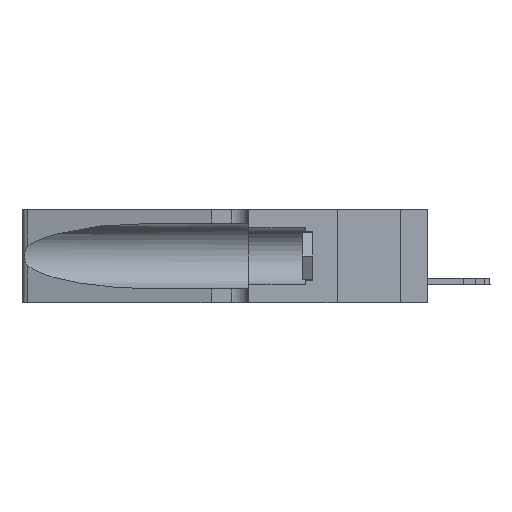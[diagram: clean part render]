
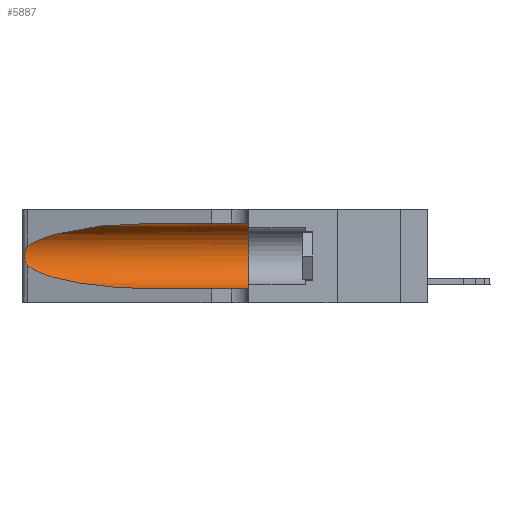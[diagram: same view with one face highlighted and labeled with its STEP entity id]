
A CAD part, left-side view. The second image highlights one B-rep face of the part: STEP entity #5887.
In plain terms, the highlighted cylindrical face has radius 3.308 mm (diameter 6.617 mm), a partial arc.
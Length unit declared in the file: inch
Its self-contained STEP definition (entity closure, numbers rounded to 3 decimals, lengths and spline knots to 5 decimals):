
#443 = FACE_OUTER_BOUND ( 'NONE', #18320, .T. ) ;
#533 = B_SPLINE_CURVE_WITH_KNOTS ( 'NONE', 3,
 ( #10524, #19248, #7877, #2828, #20661, #9650, #4468, #19108, #3426, #19643, #11725, #555, #16624, #3634 ),
 .UNSPECIFIED., .F., .F.,
 ( 4, 2, 2, 2, 2, 2, 4 ),
 ( 0., 0.00027, 0.00053, 0.00107, 0.0016, 0.00187, 0.00214 ),
 .UNSPECIFIED. ) ;
#555 = CARTESIAN_POINT ( 'NONE',  ( 0.25639, 1.23186, 0.15144 ) ) ;
#706 = CARTESIAN_POINT ( 'NONE',  ( 0.1305, 0.35, 0.185 ) ) ;
#826 = CARTESIAN_POINT ( 'NONE',  ( 0.1305, 0.72297, 0.05475 ) ) ;
#1690 = CIRCLE ( 'NONE', #1766, 0.13025 ) ;
#1766 = AXIS2_PLACEMENT_3D ( 'NONE', #706, #6352, #19618 ) ;
#1931 = LINE ( 'NONE', #5528, #7491 ) ;
#2828 = CARTESIAN_POINT ( 'NONE',  ( 0.25787, 1.23484, 0.2124 ) ) ;
#3426 = CARTESIAN_POINT ( 'NONE',  ( 0.26017, 1.23833, 0.17102 ) ) ;
#3464 = LINE ( 'NONE', #11767, #13092 ) ;
#3634 = CARTESIAN_POINT ( 'NONE',  ( 0.25487, 1.22718, 0.14631 ) ) ;
#3800 = EDGE_CURVE ( 'NONE', #15225, #18798, #4945, .T. ) ;
#4468 = CARTESIAN_POINT ( 'NONE',  ( 0.26075, 1.23896, 0.19203 ) ) ;
#4945 =( BOUNDED_CURVE ( )  B_SPLINE_CURVE ( 3, ( #10386, #12267, #8804, #20028 ),
 .UNSPECIFIED., .F., .F. ) 
 B_SPLINE_CURVE_WITH_KNOTS ( ( 4, 4 ),
 ( 1.5708, 2.84003 ),
 .UNSPECIFIED. ) 
 CURVE ( )  GEOMETRIC_REPRESENTATION_ITEM ( )  RATIONAL_B_SPLINE_CURVE ( ( 1., 0.87, 0.87, 1. ) ) 
 REPRESENTATION_ITEM ( '' )  );
#5042 = EDGE_CURVE ( 'NONE', #9095, #7832, #3464, .T. ) ;
#5292 = CARTESIAN_POINT ( 'NONE',  ( 0.1305, 0.35, 0.31525 ) ) ;
#5484 = CARTESIAN_POINT ( 'NONE',  ( 0.2373, 1.15595, 0.08982 ) ) ;
#5528 = CARTESIAN_POINT ( 'NONE',  ( 0.1305, 1.61858, 0.31525 ) ) ;
#5887 = ADVANCED_FACE ( 'NONE', ( #443 ), #19119, .F. ) ;
#6148 = CARTESIAN_POINT ( 'NONE',  ( 0.1305, 0.72297, 0.05475 ) ) ;
#6352 = DIRECTION ( 'NONE',  ( 0., 1., 0. ) ) ;
#6670 = CARTESIAN_POINT ( 'NONE',  ( 0.1305, 0.72297, 0.31525 ) ) ;
#6709 = EDGE_CURVE ( 'NONE', #20829, #7832, #1690, .T. ) ;
#7491 = VECTOR ( 'NONE', #8857, 39.37008 ) ;
#7815 = EDGE_CURVE ( 'NONE', #18853, #9095, #18726, .T. ) ;
#7832 = VERTEX_POINT ( 'NONE', #10308 ) ;
#7877 = CARTESIAN_POINT ( 'NONE',  ( 0.25639, 1.23184, 0.21858 ) ) ;
#8794 = AXIS2_PLACEMENT_3D ( 'NONE', #15442, #9673, #17578 ) ;
#8804 = CARTESIAN_POINT ( 'NONE',  ( 0.2373, 1.15595, 0.28018 ) ) ;
#8810 = CARTESIAN_POINT ( 'NONE',  ( 0.18966, 0.96281, 0.05475 ) ) ;
#8857 = DIRECTION ( 'NONE',  ( 0., -1., 0. ) ) ;
#9095 = VERTEX_POINT ( 'NONE', #6148 ) ;
#9650 = CARTESIAN_POINT ( 'NONE',  ( 0.26018, 1.23835, 0.19895 ) ) ;
#9673 = DIRECTION ( 'NONE',  ( 0., -1., 0. ) ) ;
#9890 = ORIENTED_EDGE ( 'NONE', *, *, #14328, .F. ) ;
#10308 = CARTESIAN_POINT ( 'NONE',  ( 0.1305, 0.35, 0.05475 ) ) ;
#10386 = CARTESIAN_POINT ( 'NONE',  ( 0.1305, 0.72297, 0.31525 ) ) ;
#10524 = CARTESIAN_POINT ( 'NONE',  ( 0.25487, 1.22718, 0.22369 ) ) ;
#11725 = CARTESIAN_POINT ( 'NONE',  ( 0.25789, 1.23486, 0.15765 ) ) ;
#11767 = CARTESIAN_POINT ( 'NONE',  ( 0.1305, 1.61858, 0.05475 ) ) ;
#12267 = CARTESIAN_POINT ( 'NONE',  ( 0.18966, 0.96281, 0.31525 ) ) ;
#13092 = VECTOR ( 'NONE', #14432, 39.37008 ) ;
#13213 = ORIENTED_EDGE ( 'NONE', *, *, #18365, .T. ) ;
#14328 = EDGE_CURVE ( 'NONE', #15225, #20829, #1931, .T. ) ;
#14432 = DIRECTION ( 'NONE',  ( 0., -1., 0. ) ) ;
#15127 = CARTESIAN_POINT ( 'NONE',  ( 0.25487, 1.22718, 0.14631 ) ) ;
#15225 = VERTEX_POINT ( 'NONE', #6670 ) ;
#15442 = CARTESIAN_POINT ( 'NONE',  ( 0.1305, 1.61858, 0.185 ) ) ;
#15973 = ORIENTED_EDGE ( 'NONE', *, *, #5042, .T. ) ;
#16624 = CARTESIAN_POINT ( 'NONE',  ( 0.25555, 1.22993, 0.14849 ) ) ;
#16942 = CARTESIAN_POINT ( 'NONE',  ( 0.25487, 1.22718, 0.14631 ) ) ;
#17561 = ORIENTED_EDGE ( 'NONE', *, *, #6709, .F. ) ;
#17578 = DIRECTION ( 'NONE',  ( 0., 0., -1. ) ) ;
#17781 = CARTESIAN_POINT ( 'NONE',  ( 0.25487, 1.22718, 0.22369 ) ) ;
#17949 = ORIENTED_EDGE ( 'NONE', *, *, #3800, .T. ) ;
#18320 = EDGE_LOOP ( 'NONE', ( #17949, #13213, #18701, #15973, #17561, #9890 ) ) ;
#18365 = EDGE_CURVE ( 'NONE', #18798, #18853, #533, .T. ) ;
#18701 = ORIENTED_EDGE ( 'NONE', *, *, #7815, .T. ) ;
#18726 =( BOUNDED_CURVE ( )  B_SPLINE_CURVE ( 3, ( #15127, #5484, #8810, #826 ),
 .UNSPECIFIED., .F., .T. ) 
 B_SPLINE_CURVE_WITH_KNOTS ( ( 4, 4 ),
 ( 3.44316, 4.71239 ),
 .UNSPECIFIED. ) 
 CURVE ( )  GEOMETRIC_REPRESENTATION_ITEM ( )  RATIONAL_B_SPLINE_CURVE ( ( 1., 0.87, 0.87, 1. ) ) 
 REPRESENTATION_ITEM ( '' )  );
#18798 = VERTEX_POINT ( 'NONE', #17781 ) ;
#18853 = VERTEX_POINT ( 'NONE', #16942 ) ;
#19108 = CARTESIAN_POINT ( 'NONE',  ( 0.26075, 1.23896, 0.178 ) ) ;
#19119 = CYLINDRICAL_SURFACE ( 'NONE', #8794, 0.13025 ) ;
#19248 = CARTESIAN_POINT ( 'NONE',  ( 0.25555, 1.22994, 0.2215 ) ) ;
#19618 = DIRECTION ( 'NONE',  ( 0., 0., 1. ) ) ;
#19643 = CARTESIAN_POINT ( 'NONE',  ( 0.25856, 1.23593, 0.16098 ) ) ;
#20028 = CARTESIAN_POINT ( 'NONE',  ( 0.25487, 1.22718, 0.22369 ) ) ;
#20661 = CARTESIAN_POINT ( 'NONE',  ( 0.25854, 1.2359, 0.20912 ) ) ;
#20829 = VERTEX_POINT ( 'NONE', #5292 ) ;
